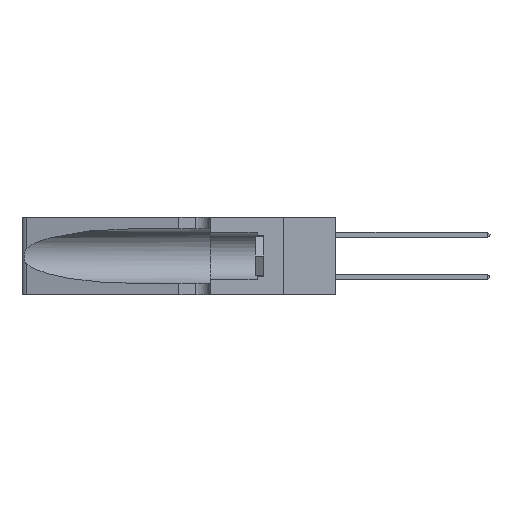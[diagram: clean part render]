
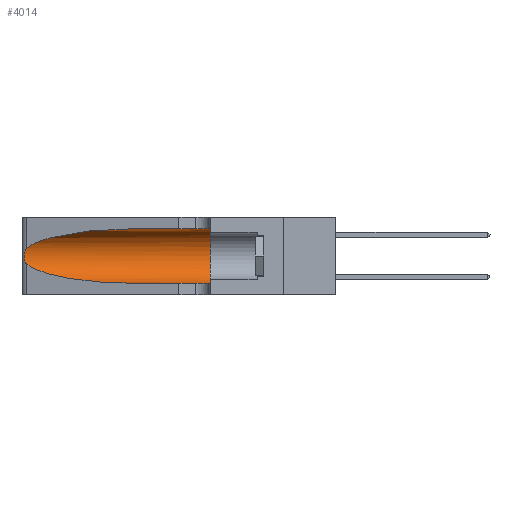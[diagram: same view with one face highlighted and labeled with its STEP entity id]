
A CAD part, left-side view. The second image highlights one B-rep face of the part: STEP entity #4014.
In plain terms, the highlighted cylindrical face has radius 3.308 mm (diameter 6.617 mm), a partial arc.
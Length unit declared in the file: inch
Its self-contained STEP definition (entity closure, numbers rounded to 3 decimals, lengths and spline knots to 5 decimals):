
#224 = DIRECTION ( 'NONE',  ( 0., -1., 0. ) ) ;
#1142 = EDGE_CURVE ( 'NONE', #5565, #11359, #8910, .T. ) ;
#2505 = VERTEX_POINT ( 'NONE', #17318 ) ;
#3292 = CYLINDRICAL_SURFACE ( 'NONE', #20806, 0.13025 ) ;
#3411 = DIRECTION ( 'NONE',  ( 0., 1., 0. ) ) ;
#3636 = CARTESIAN_POINT ( 'NONE',  ( 0.1305, 0.35, 0.05475 ) ) ;
#4014 = ADVANCED_FACE ( 'NONE', ( #4875 ), #3292, .F. ) ;
#4875 = FACE_OUTER_BOUND ( 'NONE', #29044, .T. ) ;
#5152 = CARTESIAN_POINT ( 'NONE',  ( 0.1305, 0.72297, 0.31525 ) ) ;
#5565 = VERTEX_POINT ( 'NONE', #9941 ) ;
#6023 = CARTESIAN_POINT ( 'NONE',  ( 0.25487, 1.22718, 0.14631 ) ) ;
#6124 = CARTESIAN_POINT ( 'NONE',  ( 0.25854, 1.2359, 0.20912 ) ) ;
#6789 = CARTESIAN_POINT ( 'NONE',  ( 0.1305, 1.61858, 0.05475 ) ) ;
#7309 = CARTESIAN_POINT ( 'NONE',  ( 0.2373, 1.15595, 0.28018 ) ) ;
#8244 = CARTESIAN_POINT ( 'NONE',  ( 0.26017, 1.23833, 0.17102 ) ) ;
#8408 = VECTOR ( 'NONE', #224, 39.37008 ) ;
#8529 = EDGE_CURVE ( 'NONE', #31164, #24140, #16303, .T. ) ;
#8539 = CARTESIAN_POINT ( 'NONE',  ( 0.2373, 1.15595, 0.08982 ) ) ;
#8821 = CARTESIAN_POINT ( 'NONE',  ( 0.26075, 1.23896, 0.178 ) ) ;
#8910 = CIRCLE ( 'NONE', #31914, 0.13025 ) ;
#9147 = CARTESIAN_POINT ( 'NONE',  ( 0.1305, 0.72297, 0.05475 ) ) ;
#9941 = CARTESIAN_POINT ( 'NONE',  ( 0.1305, 0.35, 0.31525 ) ) ;
#10076 = CARTESIAN_POINT ( 'NONE',  ( 0.1305, 1.61858, 0.185 ) ) ;
#10162 = CARTESIAN_POINT ( 'NONE',  ( 0.1305, 0.72297, 0.31525 ) ) ;
#10518 = ORIENTED_EDGE ( 'NONE', *, *, #10744, .T. ) ;
#10519 =( BOUNDED_CURVE ( )  B_SPLINE_CURVE ( 3, ( #5152, #16921, #7309, #24873 ),
 .UNSPECIFIED., .F., .F. ) 
 B_SPLINE_CURVE_WITH_KNOTS ( ( 4, 4 ),
 ( 1.5708, 2.84003 ),
 .UNSPECIFIED. ) 
 CURVE ( )  GEOMETRIC_REPRESENTATION_ITEM ( )  RATIONAL_B_SPLINE_CURVE ( ( 1., 0.87, 0.87, 1. ) ) 
 REPRESENTATION_ITEM ( '' )  );
#10586 = CARTESIAN_POINT ( 'NONE',  ( 0.25789, 1.23486, 0.15765 ) ) ;
#10744 = EDGE_CURVE ( 'NONE', #2505, #31164, #15892, .T. ) ;
#10809 = CARTESIAN_POINT ( 'NONE',  ( 0.25639, 1.23186, 0.15144 ) ) ;
#10923 = ORIENTED_EDGE ( 'NONE', *, *, #11707, .T. ) ;
#11359 = VERTEX_POINT ( 'NONE', #3636 ) ;
#11707 = EDGE_CURVE ( 'NONE', #21799, #2505, #10519, .T. ) ;
#12719 = DIRECTION ( 'NONE',  ( 0., 0., -1. ) ) ;
#12797 = ORIENTED_EDGE ( 'NONE', *, *, #1142, .F. ) ;
#12811 = CARTESIAN_POINT ( 'NONE',  ( 0.26075, 1.23896, 0.19203 ) ) ;
#14898 = EDGE_CURVE ( 'NONE', #21799, #5565, #29756, .T. ) ;
#15562 = CARTESIAN_POINT ( 'NONE',  ( 0.25856, 1.23593, 0.16098 ) ) ;
#15892 = B_SPLINE_CURVE_WITH_KNOTS ( 'NONE', 3,
 ( #25731, #15930, #21591, #20553, #6124, #27094, #12811, #8821, #8244, #15562, #10586, #10809, #18051, #30751 ),
 .UNSPECIFIED., .F., .F.,
 ( 4, 2, 2, 2, 2, 2, 4 ),
 ( 0., 0.00027, 0.00053, 0.00107, 0.0016, 0.00187, 0.00214 ),
 .UNSPECIFIED. ) ;
#15930 = CARTESIAN_POINT ( 'NONE',  ( 0.25555, 1.22994, 0.2215 ) ) ;
#16303 =( BOUNDED_CURVE ( )  B_SPLINE_CURVE ( 3, ( #30933, #8539, #26109, #29094 ),
 .UNSPECIFIED., .F., .F. ) 
 B_SPLINE_CURVE_WITH_KNOTS ( ( 4, 4 ),
 ( 3.44316, 4.71239 ),
 .UNSPECIFIED. ) 
 CURVE ( )  GEOMETRIC_REPRESENTATION_ITEM ( )  RATIONAL_B_SPLINE_CURVE ( ( 1., 0.87, 0.87, 1. ) ) 
 REPRESENTATION_ITEM ( '' )  );
#16921 = CARTESIAN_POINT ( 'NONE',  ( 0.18966, 0.96281, 0.31525 ) ) ;
#17318 = CARTESIAN_POINT ( 'NONE',  ( 0.25487, 1.22718, 0.22369 ) ) ;
#17431 = LINE ( 'NONE', #6789, #8408 ) ;
#17981 = EDGE_CURVE ( 'NONE', #24140, #11359, #17431, .T. ) ;
#18051 = CARTESIAN_POINT ( 'NONE',  ( 0.25555, 1.22993, 0.14849 ) ) ;
#18241 = CARTESIAN_POINT ( 'NONE',  ( 0.1305, 0.35, 0.185 ) ) ;
#19056 = CARTESIAN_POINT ( 'NONE',  ( 0.1305, 1.61858, 0.31525 ) ) ;
#19597 = VECTOR ( 'NONE', #31654, 39.37008 ) ;
#20553 = CARTESIAN_POINT ( 'NONE',  ( 0.25787, 1.23484, 0.2124 ) ) ;
#20806 = AXIS2_PLACEMENT_3D ( 'NONE', #10076, #27518, #12719 ) ;
#21109 = DIRECTION ( 'NONE',  ( 0., 0., 1. ) ) ;
#21591 = CARTESIAN_POINT ( 'NONE',  ( 0.25639, 1.23184, 0.21858 ) ) ;
#21799 = VERTEX_POINT ( 'NONE', #10162 ) ;
#23935 = ORIENTED_EDGE ( 'NONE', *, *, #17981, .T. ) ;
#24140 = VERTEX_POINT ( 'NONE', #9147 ) ;
#24873 = CARTESIAN_POINT ( 'NONE',  ( 0.25487, 1.22718, 0.22369 ) ) ;
#25731 = CARTESIAN_POINT ( 'NONE',  ( 0.25487, 1.22718, 0.22369 ) ) ;
#26109 = CARTESIAN_POINT ( 'NONE',  ( 0.18966, 0.96281, 0.05475 ) ) ;
#27094 = CARTESIAN_POINT ( 'NONE',  ( 0.26018, 1.23835, 0.19895 ) ) ;
#27518 = DIRECTION ( 'NONE',  ( 0., -1., 0. ) ) ;
#28617 = ORIENTED_EDGE ( 'NONE', *, *, #14898, .F. ) ;
#29044 = EDGE_LOOP ( 'NONE', ( #10923, #10518, #31787, #23935, #12797, #28617 ) ) ;
#29094 = CARTESIAN_POINT ( 'NONE',  ( 0.1305, 0.72297, 0.05475 ) ) ;
#29756 = LINE ( 'NONE', #19056, #19597 ) ;
#30751 = CARTESIAN_POINT ( 'NONE',  ( 0.25487, 1.22718, 0.14631 ) ) ;
#30933 = CARTESIAN_POINT ( 'NONE',  ( 0.25487, 1.22718, 0.14631 ) ) ;
#31164 = VERTEX_POINT ( 'NONE', #6023 ) ;
#31654 = DIRECTION ( 'NONE',  ( 0., -1., 0. ) ) ;
#31787 = ORIENTED_EDGE ( 'NONE', *, *, #8529, .T. ) ;
#31914 = AXIS2_PLACEMENT_3D ( 'NONE', #18241, #3411, #21109 ) ;
